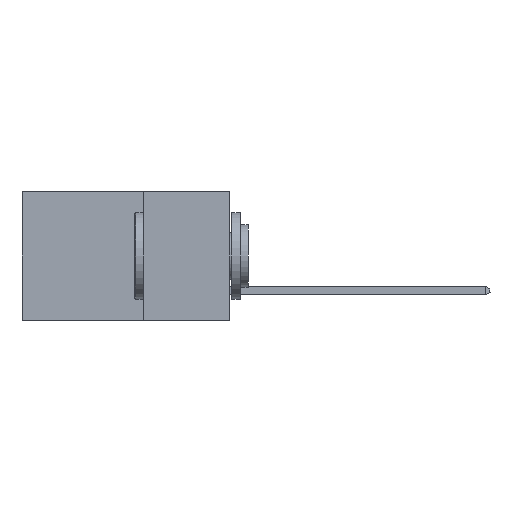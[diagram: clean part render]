
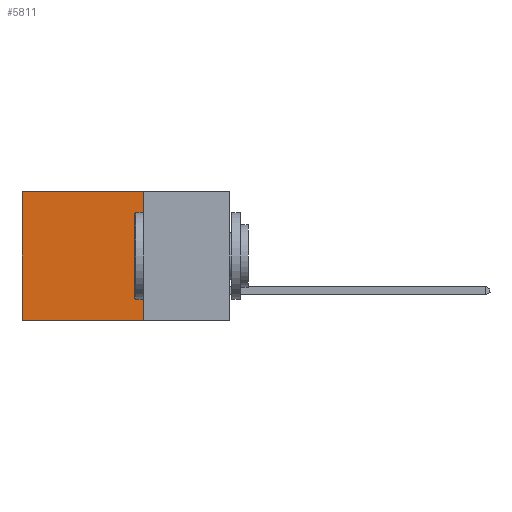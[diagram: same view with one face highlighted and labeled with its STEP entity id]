
A CAD part, left-side view. The second image highlights one B-rep face of the part: STEP entity #5811.
In plain terms, the highlighted planar face has unit normal (-1, 0, 0).
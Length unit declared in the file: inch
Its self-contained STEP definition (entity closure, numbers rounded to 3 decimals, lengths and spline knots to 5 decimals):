
#806 = CARTESIAN_POINT ( 'NONE',  ( 0.298, 0.6, 0. ) ) ;
#1171 = VECTOR ( 'NONE', #2410, 39.37008 ) ;
#1237 = PLANE ( 'NONE',  #9799 ) ;
#2027 = EDGE_CURVE ( 'NONE', #6812, #8897, #7680, .T. ) ;
#2146 = DIRECTION ( 'NONE',  ( 1., 0., 0. ) ) ;
#2323 = CARTESIAN_POINT ( 'NONE',  ( 0.298, 0.25, 0. ) ) ;
#2410 = DIRECTION ( 'NONE',  ( 0., 0., -1. ) ) ;
#4130 = CARTESIAN_POINT ( 'NONE',  ( 0.298, 0.6, 0. ) ) ;
#4710 = ORIENTED_EDGE ( 'NONE', *, *, #7673, .F. ) ;
#4771 = EDGE_CURVE ( 'NONE', #10488, #9888, #5740, .T. ) ;
#5198 = CARTESIAN_POINT ( 'NONE',  ( 0.298, 0.25, 0. ) ) ;
#5325 = VECTOR ( 'NONE', #7363, 39.37008 ) ;
#5384 = CARTESIAN_POINT ( 'NONE',  ( 0.298, 0.6, -0.37 ) ) ;
#5549 = LINE ( 'NONE', #2323, #6901 ) ;
#5740 = LINE ( 'NONE', #9095, #5325 ) ;
#5811 = ADVANCED_FACE ( 'NONE', ( #9987 ), #1237, .F. ) ;
#5976 = LINE ( 'NONE', #4130, #1171 ) ;
#6299 = ORIENTED_EDGE ( 'NONE', *, *, #7215, .T. ) ;
#6353 = DIRECTION ( 'NONE',  ( 0., 0., -1. ) ) ;
#6479 = VECTOR ( 'NONE', #10418, 39.37008 ) ;
#6544 = ORIENTED_EDGE ( 'NONE', *, *, #4771, .T. ) ;
#6777 = CARTESIAN_POINT ( 'NONE',  ( 0.298, 0.25, -0.37 ) ) ;
#6812 = VERTEX_POINT ( 'NONE', #6777 ) ;
#6901 = VECTOR ( 'NONE', #9956, 39.37008 ) ;
#7215 = EDGE_CURVE ( 'NONE', #9888, #8897, #5976, .T. ) ;
#7363 = DIRECTION ( 'NONE',  ( 0., 1., 0. ) ) ;
#7673 = EDGE_CURVE ( 'NONE', #10488, #6812, #5549, .T. ) ;
#7680 = LINE ( 'NONE', #8948, #6479 ) ;
#8897 = VERTEX_POINT ( 'NONE', #5384 ) ;
#8948 = CARTESIAN_POINT ( 'NONE',  ( 0.298, 0.25, -0.37 ) ) ;
#8970 = ORIENTED_EDGE ( 'NONE', *, *, #2027, .F. ) ;
#9095 = CARTESIAN_POINT ( 'NONE',  ( 0.298, 0.25, 0. ) ) ;
#9799 = AXIS2_PLACEMENT_3D ( 'NONE', #10576, #2146, #6353 ) ;
#9888 = VERTEX_POINT ( 'NONE', #806 ) ;
#9956 = DIRECTION ( 'NONE',  ( 0., 0., -1. ) ) ;
#9987 = FACE_OUTER_BOUND ( 'NONE', #10854, .T. ) ;
#10418 = DIRECTION ( 'NONE',  ( 0., 1., 0. ) ) ;
#10488 = VERTEX_POINT ( 'NONE', #5198 ) ;
#10576 = CARTESIAN_POINT ( 'NONE',  ( 0.298, 0.25, 0. ) ) ;
#10854 = EDGE_LOOP ( 'NONE', ( #6299, #8970, #4710, #6544 ) ) ;
